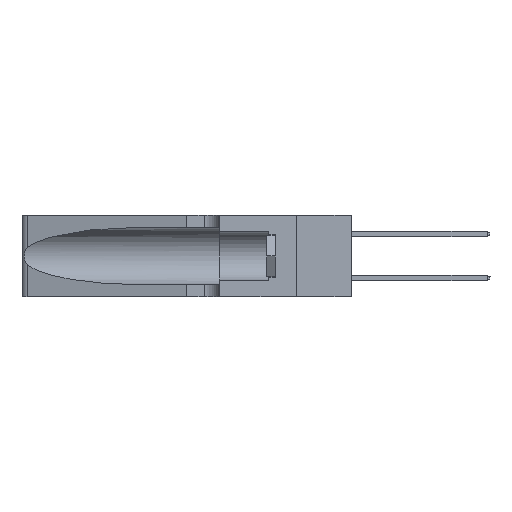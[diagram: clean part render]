
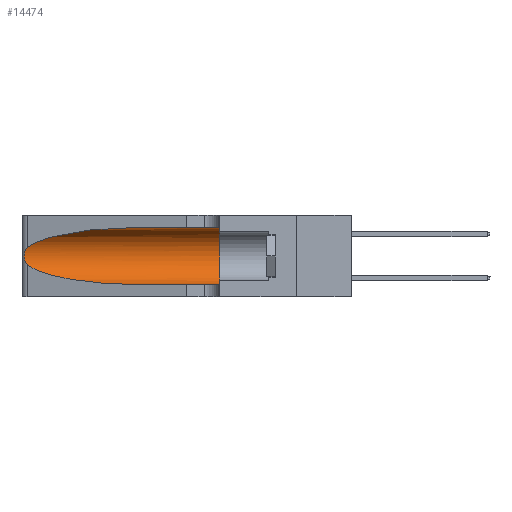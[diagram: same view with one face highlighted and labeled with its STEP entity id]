
A CAD part, left-side view. The second image highlights one B-rep face of the part: STEP entity #14474.
In plain terms, the highlighted cylindrical face has radius 3.308 mm (diameter 6.617 mm), a partial arc.
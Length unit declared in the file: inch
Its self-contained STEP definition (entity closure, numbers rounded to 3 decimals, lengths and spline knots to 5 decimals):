
#3183 = CARTESIAN_POINT ( 'NONE',  ( 0.25854, 1.2359, 0.20912 ) ) ;
#4150 = LINE ( 'NONE', #13629, #25226 ) ;
#4384 = VECTOR ( 'NONE', #23002, 39.37008 ) ;
#4930 = VERTEX_POINT ( 'NONE', #31497 ) ;
#5261 = EDGE_CURVE ( 'NONE', #15648, #41715, #28598, .T. ) ;
#5831 = CARTESIAN_POINT ( 'NONE',  ( 0.1305, 1.61858, 0.05475 ) ) ;
#6381 = VERTEX_POINT ( 'NONE', #26334 ) ;
#6544 = DIRECTION ( 'NONE',  ( 0., -1., 0. ) ) ;
#6875 = CARTESIAN_POINT ( 'NONE',  ( 0.26075, 1.23896, 0.178 ) ) ;
#6985 = CARTESIAN_POINT ( 'NONE',  ( 0.1305, 0.72297, 0.05475 ) ) ;
#7209 = CARTESIAN_POINT ( 'NONE',  ( 0.1305, 0.72297, 0.31525 ) ) ;
#7560 = ORIENTED_EDGE ( 'NONE', *, *, #28690, .T. ) ;
#7610 = CARTESIAN_POINT ( 'NONE',  ( 0.1305, 0.35, 0.31525 ) ) ;
#8277 = ORIENTED_EDGE ( 'NONE', *, *, #5261, .T. ) ;
#8450 = EDGE_LOOP ( 'NONE', ( #7560, #21956, #41693, #8277, #16900, #35706 ) ) ;
#8957 = CYLINDRICAL_SURFACE ( 'NONE', #42247, 0.13025 ) ;
#10224 = CARTESIAN_POINT ( 'NONE',  ( 0.18966, 0.96281, 0.05475 ) ) ;
#10572 = CARTESIAN_POINT ( 'NONE',  ( 0.2373, 1.15595, 0.28018 ) ) ;
#13065 = EDGE_CURVE ( 'NONE', #35439, #6381, #23840, .T. ) ;
#13488 = CARTESIAN_POINT ( 'NONE',  ( 0.26075, 1.23896, 0.19203 ) ) ;
#13629 = CARTESIAN_POINT ( 'NONE',  ( 0.1305, 1.61858, 0.31525 ) ) ;
#14468 = EDGE_CURVE ( 'NONE', #6381, #15648, #16065, .T. ) ;
#14474 = ADVANCED_FACE ( 'NONE', ( #17325 ), #8957, .F. ) ;
#14866 = EDGE_CURVE ( 'NONE', #4930, #41314, #4150, .T. ) ;
#15119 = DIRECTION ( 'NONE',  ( 0., -1., 0. ) ) ;
#15270 =( BOUNDED_CURVE ( )  B_SPLINE_CURVE ( 3, ( #7209, #21012, #10572, #27434 ),
 .UNSPECIFIED., .F., .T. ) 
 B_SPLINE_CURVE_WITH_KNOTS ( ( 4, 4 ),
 ( 1.5708, 2.84003 ),
 .UNSPECIFIED. ) 
 CURVE ( )  GEOMETRIC_REPRESENTATION_ITEM ( )  RATIONAL_B_SPLINE_CURVE ( ( 1., 0.87, 0.87, 1. ) ) 
 REPRESENTATION_ITEM ( '' )  );
#15648 = VERTEX_POINT ( 'NONE', #32988 ) ;
#16065 =( BOUNDED_CURVE ( )  B_SPLINE_CURVE ( 3, ( #29798, #17715, #10224, #6985 ),
 .UNSPECIFIED., .F., .F. ) 
 B_SPLINE_CURVE_WITH_KNOTS ( ( 4, 4 ),
 ( 3.44316, 4.71239 ),
 .UNSPECIFIED. ) 
 CURVE ( )  GEOMETRIC_REPRESENTATION_ITEM ( )  RATIONAL_B_SPLINE_CURVE ( ( 1., 0.87, 0.87, 1. ) ) 
 REPRESENTATION_ITEM ( '' )  );
#16403 = CARTESIAN_POINT ( 'NONE',  ( 0.1305, 1.61858, 0.185 ) ) ;
#16714 = CARTESIAN_POINT ( 'NONE',  ( 0.25789, 1.23486, 0.15765 ) ) ;
#16900 = ORIENTED_EDGE ( 'NONE', *, *, #23637, .F. ) ;
#17325 = FACE_OUTER_BOUND ( 'NONE', #8450, .T. ) ;
#17715 = CARTESIAN_POINT ( 'NONE',  ( 0.2373, 1.15595, 0.08982 ) ) ;
#18473 = CARTESIAN_POINT ( 'NONE',  ( 0.1305, 0.35, 0.05475 ) ) ;
#18716 = CARTESIAN_POINT ( 'NONE',  ( 0.1305, 0.35, 0.185 ) ) ;
#19916 = DIRECTION ( 'NONE',  ( 0., 0., -1. ) ) ;
#20518 = CARTESIAN_POINT ( 'NONE',  ( 0.26018, 1.23835, 0.19895 ) ) ;
#21012 = CARTESIAN_POINT ( 'NONE',  ( 0.18966, 0.96281, 0.31525 ) ) ;
#21956 = ORIENTED_EDGE ( 'NONE', *, *, #13065, .T. ) ;
#23002 = DIRECTION ( 'NONE',  ( 0., -1., 0. ) ) ;
#23471 = CARTESIAN_POINT ( 'NONE',  ( 0.25639, 1.23186, 0.15144 ) ) ;
#23637 = EDGE_CURVE ( 'NONE', #41314, #41715, #27499, .T. ) ;
#23840 = B_SPLINE_CURVE_WITH_KNOTS ( 'NONE', 3,
 ( #26991, #26704, #43480, #40661, #3183, #20518, #13488, #6875, #30098, #36874, #16714, #23471, #30379, #26845 ),
 .UNSPECIFIED., .F., .F.,
 ( 4, 2, 2, 2, 2, 2, 4 ),
 ( 0., 0.00027, 0.00053, 0.00107, 0.0016, 0.00187, 0.00214 ),
 .UNSPECIFIED. ) ;
#25048 = DIRECTION ( 'NONE',  ( 0., 0., 1. ) ) ;
#25226 = VECTOR ( 'NONE', #15119, 39.37008 ) ;
#26334 = CARTESIAN_POINT ( 'NONE',  ( 0.25487, 1.22718, 0.14631 ) ) ;
#26704 = CARTESIAN_POINT ( 'NONE',  ( 0.25555, 1.22994, 0.2215 ) ) ;
#26845 = CARTESIAN_POINT ( 'NONE',  ( 0.25487, 1.22718, 0.14631 ) ) ;
#26991 = CARTESIAN_POINT ( 'NONE',  ( 0.25487, 1.22718, 0.22369 ) ) ;
#27434 = CARTESIAN_POINT ( 'NONE',  ( 0.25487, 1.22718, 0.22369 ) ) ;
#27499 = CIRCLE ( 'NONE', #39646, 0.13025 ) ;
#27687 = CARTESIAN_POINT ( 'NONE',  ( 0.25487, 1.22718, 0.22369 ) ) ;
#28598 = LINE ( 'NONE', #5831, #4384 ) ;
#28690 = EDGE_CURVE ( 'NONE', #4930, #35439, #15270, .T. ) ;
#29798 = CARTESIAN_POINT ( 'NONE',  ( 0.25487, 1.22718, 0.14631 ) ) ;
#30098 = CARTESIAN_POINT ( 'NONE',  ( 0.26017, 1.23833, 0.17102 ) ) ;
#30379 = CARTESIAN_POINT ( 'NONE',  ( 0.25555, 1.22993, 0.14849 ) ) ;
#31497 = CARTESIAN_POINT ( 'NONE',  ( 0.1305, 0.72297, 0.31525 ) ) ;
#31958 = DIRECTION ( 'NONE',  ( 0., 1., 0. ) ) ;
#32988 = CARTESIAN_POINT ( 'NONE',  ( 0.1305, 0.72297, 0.05475 ) ) ;
#35439 = VERTEX_POINT ( 'NONE', #27687 ) ;
#35706 = ORIENTED_EDGE ( 'NONE', *, *, #14866, .F. ) ;
#36874 = CARTESIAN_POINT ( 'NONE',  ( 0.25856, 1.23593, 0.16098 ) ) ;
#39646 = AXIS2_PLACEMENT_3D ( 'NONE', #18716, #31958, #25048 ) ;
#40661 = CARTESIAN_POINT ( 'NONE',  ( 0.25787, 1.23484, 0.2124 ) ) ;
#41314 = VERTEX_POINT ( 'NONE', #7610 ) ;
#41693 = ORIENTED_EDGE ( 'NONE', *, *, #14468, .T. ) ;
#41715 = VERTEX_POINT ( 'NONE', #18473 ) ;
#42247 = AXIS2_PLACEMENT_3D ( 'NONE', #16403, #6544, #19916 ) ;
#43480 = CARTESIAN_POINT ( 'NONE',  ( 0.25639, 1.23184, 0.21858 ) ) ;
